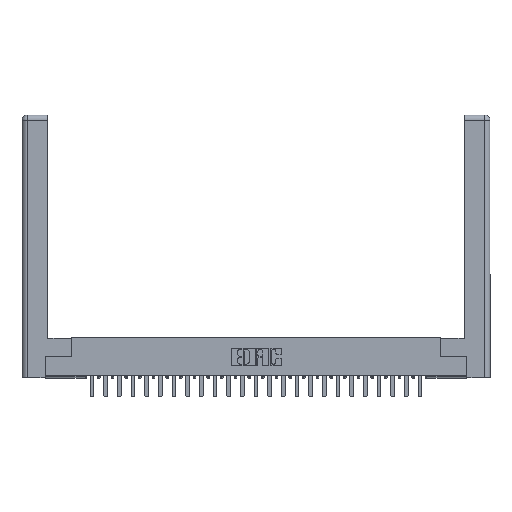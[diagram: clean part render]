
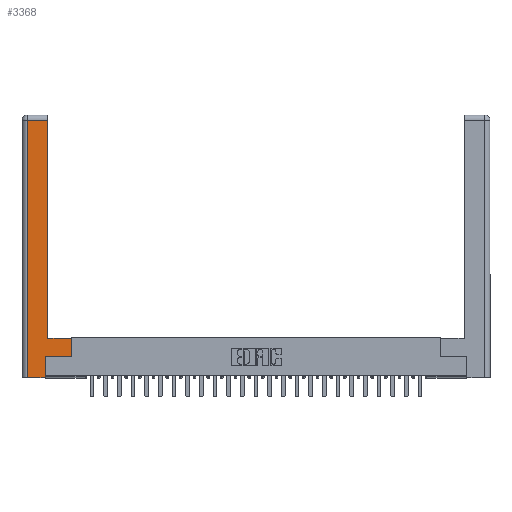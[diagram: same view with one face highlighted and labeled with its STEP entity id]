
A CAD part, top view. The second image highlights one B-rep face of the part: STEP entity #3368.
In plain terms, the highlighted planar face has unit normal (0, 0, 1).
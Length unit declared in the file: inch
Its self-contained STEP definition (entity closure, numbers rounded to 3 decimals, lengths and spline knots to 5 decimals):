
#1882 = VECTOR ( 'NONE', #10973, 39.37008 ) ;
#1940 = DIRECTION ( 'NONE',  ( 0., 1., 0. ) ) ;
#1946 = VECTOR ( 'NONE', #4651, 39.37008 ) ;
#2249 = LINE ( 'NONE', #27956, #1882 ) ;
#2403 = VECTOR ( 'NONE', #30191, 39.37008 ) ;
#2508 = CARTESIAN_POINT ( 'NONE',  ( 0.265, 0.245, 0. ) ) ;
#2601 = ORIENTED_EDGE ( 'NONE', *, *, #31352, .T. ) ;
#2612 = EDGE_CURVE ( 'NONE', #22815, #31215, #20152, .T. ) ;
#2674 = DIRECTION ( 'NONE',  ( -1., 0., 0. ) ) ;
#3179 = LINE ( 'NONE', #20092, #2403 ) ;
#3368 = ADVANCED_FACE ( 'NONE', ( #17855 ), #4098, .F. ) ;
#3465 = DIRECTION ( 'NONE',  ( 1., 0., 0. ) ) ;
#4087 = ORIENTED_EDGE ( 'NONE', *, *, #2612, .T. ) ;
#4098 = PLANE ( 'NONE',  #18900 ) ;
#4651 = DIRECTION ( 'NONE',  ( 0., 1., 0. ) ) ;
#5038 = LINE ( 'NONE', #6691, #30282 ) ;
#6150 = CARTESIAN_POINT ( 'NONE',  ( 0.295, 0.45, 0. ) ) ;
#6583 = EDGE_CURVE ( 'NONE', #28040, #24455, #2249, .T. ) ;
#6691 = CARTESIAN_POINT ( 'NONE',  ( 0.0615, 2.94, 0. ) ) ;
#6991 = CARTESIAN_POINT ( 'NONE',  ( 0.565, 0.245, 0. ) ) ;
#7734 = EDGE_CURVE ( 'NONE', #31215, #10025, #27402, .T. ) ;
#7945 = LINE ( 'NONE', #22255, #24756 ) ;
#8353 = LINE ( 'NONE', #20779, #11015 ) ;
#9529 = CARTESIAN_POINT ( 'NONE',  ( 0., 0., 0. ) ) ;
#10025 = VERTEX_POINT ( 'NONE', #16099 ) ;
#10973 = DIRECTION ( 'NONE',  ( 0., 1., 0. ) ) ;
#11015 = VECTOR ( 'NONE', #15697, 39.37008 ) ;
#11907 = CARTESIAN_POINT ( 'NONE',  ( 0.565, 0.45, 0. ) ) ;
#11992 = DIRECTION ( 'NONE',  ( -1., 0., 0. ) ) ;
#12223 = EDGE_CURVE ( 'NONE', #12379, #19078, #3179, .T. ) ;
#12379 = VERTEX_POINT ( 'NONE', #26095 ) ;
#12793 = CARTESIAN_POINT ( 'NONE',  ( 0.265, 0.245, 0. ) ) ;
#13498 = EDGE_CURVE ( 'NONE', #24455, #22556, #5038, .T. ) ;
#13503 = ORIENTED_EDGE ( 'NONE', *, *, #7734, .T. ) ;
#13558 = EDGE_CURVE ( 'NONE', #19078, #22815, #27933, .T. ) ;
#14680 = ORIENTED_EDGE ( 'NONE', *, *, #13498, .T. ) ;
#15697 = DIRECTION ( 'NONE',  ( 0., -1., 0. ) ) ;
#16099 = CARTESIAN_POINT ( 'NONE',  ( 0.565, 0.45, 0. ) ) ;
#17855 = FACE_OUTER_BOUND ( 'NONE', #30868, .T. ) ;
#18090 = ORIENTED_EDGE ( 'NONE', *, *, #31568, .T. ) ;
#18900 = AXIS2_PLACEMENT_3D ( 'NONE', #9529, #26616, #11992 ) ;
#19078 = VERTEX_POINT ( 'NONE', #21387 ) ;
#20092 = CARTESIAN_POINT ( 'NONE',  ( 0.265, 0., 0. ) ) ;
#20152 = LINE ( 'NONE', #6991, #20914 ) ;
#20779 = CARTESIAN_POINT ( 'NONE',  ( 0.0615, 0., 0. ) ) ;
#20914 = VECTOR ( 'NONE', #3465, 39.37008 ) ;
#21387 = CARTESIAN_POINT ( 'NONE',  ( 0.265, 0., 0. ) ) ;
#22255 = CARTESIAN_POINT ( 'NONE',  ( 0.295, 0.45, 0. ) ) ;
#22556 = VERTEX_POINT ( 'NONE', #26202 ) ;
#22815 = VERTEX_POINT ( 'NONE', #12793 ) ;
#24455 = VERTEX_POINT ( 'NONE', #27842 ) ;
#24756 = VECTOR ( 'NONE', #2674, 39.37008 ) ;
#24960 = CARTESIAN_POINT ( 'NONE',  ( 0.565, 0.245, 0. ) ) ;
#26095 = CARTESIAN_POINT ( 'NONE',  ( 0.0615, 0., 0. ) ) ;
#26202 = CARTESIAN_POINT ( 'NONE',  ( 0.0615, 2.94, 0. ) ) ;
#26220 = DIRECTION ( 'NONE',  ( -1., 0., 0. ) ) ;
#26521 = ORIENTED_EDGE ( 'NONE', *, *, #6583, .T. ) ;
#26616 = DIRECTION ( 'NONE',  ( 0., 0., -1. ) ) ;
#26951 = ORIENTED_EDGE ( 'NONE', *, *, #12223, .T. ) ;
#27065 = ORIENTED_EDGE ( 'NONE', *, *, #13558, .T. ) ;
#27402 = LINE ( 'NONE', #11907, #28554 ) ;
#27842 = CARTESIAN_POINT ( 'NONE',  ( 0.295, 2.94, 0. ) ) ;
#27933 = LINE ( 'NONE', #2508, #1946 ) ;
#27956 = CARTESIAN_POINT ( 'NONE',  ( 0.295, 3., 0. ) ) ;
#28040 = VERTEX_POINT ( 'NONE', #6150 ) ;
#28554 = VECTOR ( 'NONE', #1940, 39.37008 ) ;
#30191 = DIRECTION ( 'NONE',  ( 1., 0., 0. ) ) ;
#30282 = VECTOR ( 'NONE', #26220, 39.37008 ) ;
#30868 = EDGE_LOOP ( 'NONE', ( #26521, #14680, #2601, #26951, #27065, #4087, #13503, #18090 ) ) ;
#31215 = VERTEX_POINT ( 'NONE', #24960 ) ;
#31352 = EDGE_CURVE ( 'NONE', #22556, #12379, #8353, .T. ) ;
#31568 = EDGE_CURVE ( 'NONE', #10025, #28040, #7945, .T. ) ;
